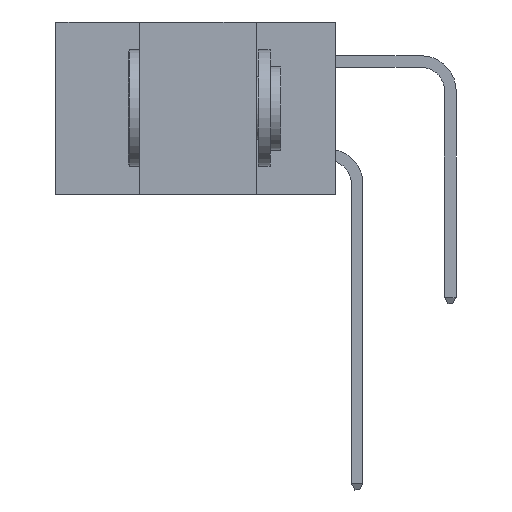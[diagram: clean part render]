
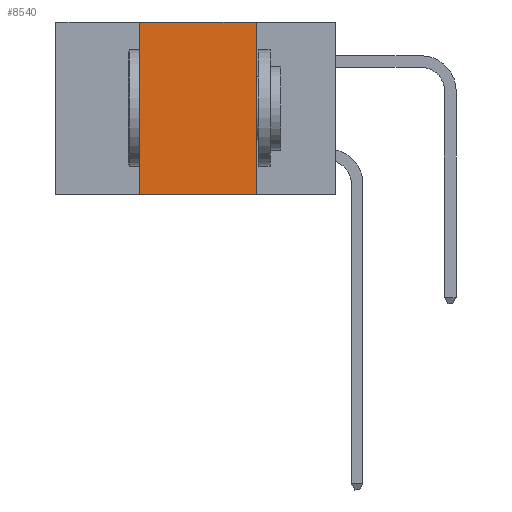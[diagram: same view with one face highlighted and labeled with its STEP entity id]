
A CAD part, left-side view. The second image highlights one B-rep face of the part: STEP entity #8540.
In plain terms, the highlighted planar face has unit normal (-1, 0, 0).
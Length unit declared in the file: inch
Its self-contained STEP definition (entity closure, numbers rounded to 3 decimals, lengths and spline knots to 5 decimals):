
#212 = ORIENTED_EDGE ( 'NONE', *, *, #30458, .T. ) ;
#294 = ORIENTED_EDGE ( 'NONE', *, *, #6235, .F. ) ;
#585 = CARTESIAN_POINT ( 'NONE',  ( 0., 0.42, -0.37 ) ) ;
#696 = VERTEX_POINT ( 'NONE', #16132 ) ;
#1145 = ORIENTED_EDGE ( 'NONE', *, *, #19034, .F. ) ;
#1191 = DIRECTION ( 'NONE',  ( 0., 0., -1. ) ) ;
#1520 = CARTESIAN_POINT ( 'NONE',  ( 0., 0.6, 0. ) ) ;
#3751 = EDGE_LOOP ( 'NONE', ( #1145, #294, #9277, #212 ) ) ;
#4029 = LINE ( 'NONE', #13736, #17607 ) ;
#5479 = PLANE ( 'NONE',  #16247 ) ;
#6235 = EDGE_CURVE ( 'NONE', #30849, #696, #13753, .T. ) ;
#6816 = CARTESIAN_POINT ( 'NONE',  ( 0., 0.42, 0. ) ) ;
#8026 = DIRECTION ( 'NONE',  ( 1., 0., 0. ) ) ;
#8540 = ADVANCED_FACE ( 'NONE', ( #11991 ), #5479, .F. ) ;
#8581 = DIRECTION ( 'NONE',  ( 0., -1., 0. ) ) ;
#9173 = CARTESIAN_POINT ( 'NONE',  ( 0., 0.17, -0.37 ) ) ;
#9277 = ORIENTED_EDGE ( 'NONE', *, *, #19675, .F. ) ;
#9528 = VECTOR ( 'NONE', #26263, 39.37008 ) ;
#11427 = VERTEX_POINT ( 'NONE', #9173 ) ;
#11757 = DIRECTION ( 'NONE',  ( 0., -1., 0. ) ) ;
#11991 = FACE_OUTER_BOUND ( 'NONE', #3751, .T. ) ;
#12959 = VECTOR ( 'NONE', #11757, 39.37008 ) ;
#13736 = CARTESIAN_POINT ( 'NONE',  ( 0., 0.6, -0.37 ) ) ;
#13753 = LINE ( 'NONE', #1520, #12959 ) ;
#13867 = CARTESIAN_POINT ( 'NONE',  ( 0., 0.17, 0. ) ) ;
#15985 = LINE ( 'NONE', #13867, #28663 ) ;
#16132 = CARTESIAN_POINT ( 'NONE',  ( 0., 0.17, 0. ) ) ;
#16186 = CARTESIAN_POINT ( 'NONE',  ( 0., 0.42, 0. ) ) ;
#16247 = AXIS2_PLACEMENT_3D ( 'NONE', #25757, #8026, #25854 ) ;
#17607 = VECTOR ( 'NONE', #8581, 39.37008 ) ;
#19034 = EDGE_CURVE ( 'NONE', #696, #11427, #15985, .T. ) ;
#19675 = EDGE_CURVE ( 'NONE', #25869, #30849, #23058, .T. ) ;
#23058 = LINE ( 'NONE', #16186, #9528 ) ;
#25757 = CARTESIAN_POINT ( 'NONE',  ( 0., 0.6, 0. ) ) ;
#25854 = DIRECTION ( 'NONE',  ( 0., 0., -1. ) ) ;
#25869 = VERTEX_POINT ( 'NONE', #585 ) ;
#26263 = DIRECTION ( 'NONE',  ( 0., 0., 1. ) ) ;
#28663 = VECTOR ( 'NONE', #1191, 39.37008 ) ;
#30458 = EDGE_CURVE ( 'NONE', #25869, #11427, #4029, .T. ) ;
#30849 = VERTEX_POINT ( 'NONE', #6816 ) ;
